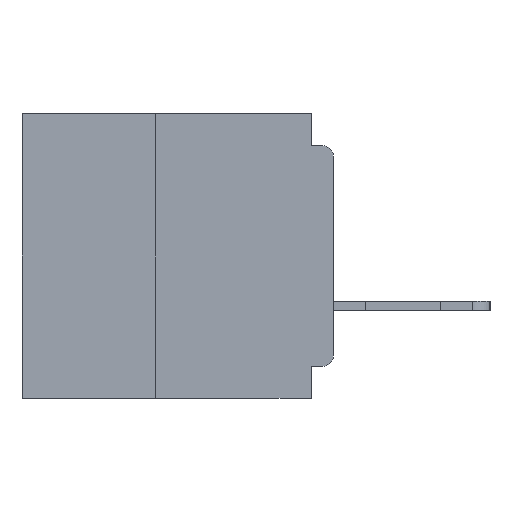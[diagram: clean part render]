
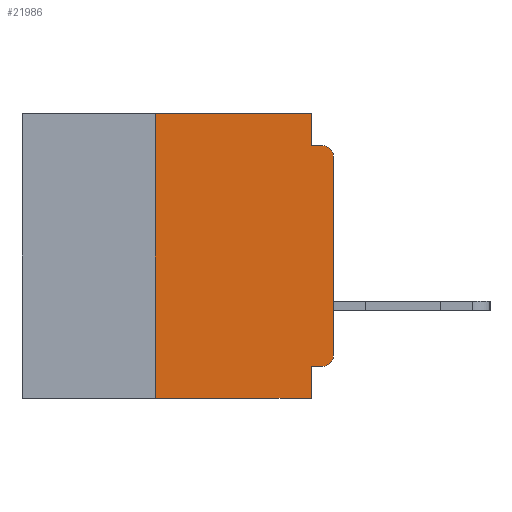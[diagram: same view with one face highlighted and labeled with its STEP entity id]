
A CAD part, left-side view. The second image highlights one B-rep face of the part: STEP entity #21986.
In plain terms, the highlighted planar face has unit normal (-1, 0, 0).
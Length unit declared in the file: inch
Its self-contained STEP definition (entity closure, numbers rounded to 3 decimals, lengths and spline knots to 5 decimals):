
#13 = DIRECTION ( 'NONE',  ( 0., -1., 0. ) ) ;
#1113 = ORIENTED_EDGE ( 'NONE', *, *, #14171, .F. ) ;
#2782 = VECTOR ( 'NONE', #36942, 39.37008 ) ;
#2877 = ORIENTED_EDGE ( 'NONE', *, *, #11118, .T. ) ;
#2984 = VECTOR ( 'NONE', #26366, 39.37008 ) ;
#3753 = EDGE_CURVE ( 'NONE', #34786, #18414, #17581, .T. ) ;
#3757 = VECTOR ( 'NONE', #10649, 39.37008 ) ;
#3830 = VERTEX_POINT ( 'NONE', #19802 ) ;
#3960 = CARTESIAN_POINT ( 'NONE',  ( 0., 0.015, -0.045 ) ) ;
#4042 = CARTESIAN_POINT ( 'NONE',  ( 0., 0.015, -0.06 ) ) ;
#4301 = VERTEX_POINT ( 'NONE', #7063 ) ;
#4696 = ORIENTED_EDGE ( 'NONE', *, *, #22352, .T. ) ;
#4764 = CARTESIAN_POINT ( 'NONE',  ( 0., 0.25, -0.4 ) ) ;
#5815 = LINE ( 'NONE', #10612, #35255 ) ;
#6314 = ORIENTED_EDGE ( 'NONE', *, *, #3753, .F. ) ;
#6870 = CARTESIAN_POINT ( 'NONE',  ( 0., 0.031, -0.355 ) ) ;
#6974 = DIRECTION ( 'NONE',  ( 0., 0., -1. ) ) ;
#7063 = CARTESIAN_POINT ( 'NONE',  ( 0., 0.25, 0. ) ) ;
#7309 = ORIENTED_EDGE ( 'NONE', *, *, #22776, .T. ) ;
#7712 = CARTESIAN_POINT ( 'NONE',  ( 0., 0., 0. ) ) ;
#7912 = CARTESIAN_POINT ( 'NONE',  ( 0., 0., -0.34 ) ) ;
#8354 = ORIENTED_EDGE ( 'NONE', *, *, #26221, .F. ) ;
#8737 = PLANE ( 'NONE',  #10878 ) ;
#8852 = DIRECTION ( 'NONE',  ( 0., 0., -1. ) ) ;
#9500 = CARTESIAN_POINT ( 'NONE',  ( 0., 0.031, -0.4 ) ) ;
#10361 = VERTEX_POINT ( 'NONE', #3960 ) ;
#10426 = CARTESIAN_POINT ( 'NONE',  ( 0., 0.437, -0.4 ) ) ;
#10612 = CARTESIAN_POINT ( 'NONE',  ( 0., 0., -0.355 ) ) ;
#10645 = EDGE_LOOP ( 'NONE', ( #7309, #30224, #21719, #6314, #16815, #1113, #2877, #22515, #8354, #4696 ) ) ;
#10649 = DIRECTION ( 'NONE',  ( 0., 0., 1. ) ) ;
#10747 = VECTOR ( 'NONE', #16616, 39.37008 ) ;
#10756 = LINE ( 'NONE', #37997, #2984 ) ;
#10878 = AXIS2_PLACEMENT_3D ( 'NONE', #20664, #26572, #8852 ) ;
#11118 = EDGE_CURVE ( 'NONE', #17870, #25017, #35366, .T. ) ;
#11690 = CARTESIAN_POINT ( 'NONE',  ( 0., 0.015, -0.34 ) ) ;
#11890 = CARTESIAN_POINT ( 'NONE',  ( 0., 0., -0.06 ) ) ;
#13748 = VECTOR ( 'NONE', #25091, 39.37008 ) ;
#13939 = VECTOR ( 'NONE', #13, 39.37008 ) ;
#14171 = EDGE_CURVE ( 'NONE', #17870, #4301, #10756, .T. ) ;
#14742 = DIRECTION ( 'NONE',  ( 0., 0., -1. ) ) ;
#15271 = EDGE_CURVE ( 'NONE', #18414, #10361, #26524, .T. ) ;
#15400 = VECTOR ( 'NONE', #33058, 39.37008 ) ;
#16616 = DIRECTION ( 'NONE',  ( 0., -1., 0. ) ) ;
#16815 = ORIENTED_EDGE ( 'NONE', *, *, #21978, .F. ) ;
#17581 = LINE ( 'NONE', #19430, #2782 ) ;
#17870 = VERTEX_POINT ( 'NONE', #4764 ) ;
#18214 = AXIS2_PLACEMENT_3D ( 'NONE', #4042, #24670, #6974 ) ;
#18414 = VERTEX_POINT ( 'NONE', #22031 ) ;
#19430 = CARTESIAN_POINT ( 'NONE',  ( 0., 0.031, 0. ) ) ;
#19489 = LINE ( 'NONE', #7712, #3757 ) ;
#19802 = CARTESIAN_POINT ( 'NONE',  ( 0., 0.015, -0.355 ) ) ;
#20148 = AXIS2_PLACEMENT_3D ( 'NONE', #11690, #32330, #14742 ) ;
#20664 = CARTESIAN_POINT ( 'NONE',  ( 0., 0.437, 0. ) ) ;
#21719 = ORIENTED_EDGE ( 'NONE', *, *, #15271, .F. ) ;
#21832 = LINE ( 'NONE', #38076, #13939 ) ;
#21978 = EDGE_CURVE ( 'NONE', #4301, #34786, #21832, .T. ) ;
#21986 = ADVANCED_FACE ( 'NONE', ( #37387 ), #8737, .F. ) ;
#22031 = CARTESIAN_POINT ( 'NONE',  ( 0., 0.031, -0.045 ) ) ;
#22352 = EDGE_CURVE ( 'NONE', #3830, #30739, #33210, .T. ) ;
#22515 = ORIENTED_EDGE ( 'NONE', *, *, #33400, .F. ) ;
#22776 = EDGE_CURVE ( 'NONE', #30739, #34752, #19489, .T. ) ;
#24098 = CARTESIAN_POINT ( 'NONE',  ( 0., 0.031, 0. ) ) ;
#24434 = CIRCLE ( 'NONE', #18214, 0.015 ) ;
#24670 = DIRECTION ( 'NONE',  ( -1., 0., 0. ) ) ;
#24757 = CARTESIAN_POINT ( 'NONE',  ( 0., 0.031, -0.4 ) ) ;
#25017 = VERTEX_POINT ( 'NONE', #24757 ) ;
#25091 = DIRECTION ( 'NONE',  ( 0., -1., 0. ) ) ;
#26221 = EDGE_CURVE ( 'NONE', #3830, #31129, #5815, .T. ) ;
#26366 = DIRECTION ( 'NONE',  ( 0., 0., 1. ) ) ;
#26524 = LINE ( 'NONE', #37135, #10747 ) ;
#26572 = DIRECTION ( 'NONE',  ( 1., 0., 0. ) ) ;
#27346 = EDGE_CURVE ( 'NONE', #34752, #10361, #24434, .T. ) ;
#28334 = DIRECTION ( 'NONE',  ( 0., 1., 0. ) ) ;
#29242 = LINE ( 'NONE', #9500, #15400 ) ;
#30224 = ORIENTED_EDGE ( 'NONE', *, *, #27346, .T. ) ;
#30739 = VERTEX_POINT ( 'NONE', #7912 ) ;
#31129 = VERTEX_POINT ( 'NONE', #6870 ) ;
#32330 = DIRECTION ( 'NONE',  ( -1., 0., 0. ) ) ;
#33058 = DIRECTION ( 'NONE',  ( 0., 0., -1. ) ) ;
#33210 = CIRCLE ( 'NONE', #20148, 0.015 ) ;
#33400 = EDGE_CURVE ( 'NONE', #31129, #25017, #29242, .T. ) ;
#34752 = VERTEX_POINT ( 'NONE', #11890 ) ;
#34786 = VERTEX_POINT ( 'NONE', #24098 ) ;
#35255 = VECTOR ( 'NONE', #28334, 39.37008 ) ;
#35366 = LINE ( 'NONE', #10426, #13748 ) ;
#36942 = DIRECTION ( 'NONE',  ( 0., 0., -1. ) ) ;
#37135 = CARTESIAN_POINT ( 'NONE',  ( 0., 0., -0.045 ) ) ;
#37387 = FACE_OUTER_BOUND ( 'NONE', #10645, .T. ) ;
#37997 = CARTESIAN_POINT ( 'NONE',  ( 0., 0.25, -0.4 ) ) ;
#38076 = CARTESIAN_POINT ( 'NONE',  ( 0., 0.437, 0. ) ) ;
